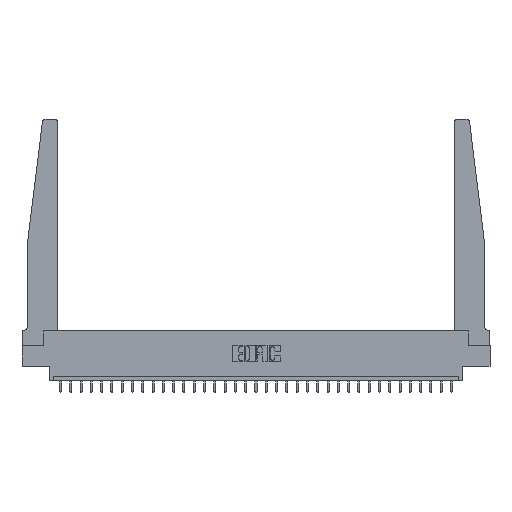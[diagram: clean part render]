
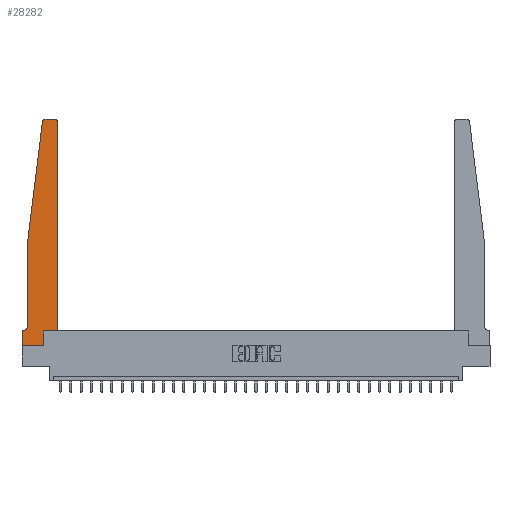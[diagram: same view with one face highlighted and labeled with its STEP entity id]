
A CAD part, top view. The second image highlights one B-rep face of the part: STEP entity #28282.
In plain terms, the highlighted planar face has unit normal (0, 0, 1).
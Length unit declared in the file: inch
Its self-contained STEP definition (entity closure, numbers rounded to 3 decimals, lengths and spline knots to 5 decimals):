
#91 = AXIS2_PLACEMENT_3D ( 'NONE', #8846, #29325, #2032 ) ;
#441 = VECTOR ( 'NONE', #27122, 39.37008 ) ;
#779 = CARTESIAN_POINT ( 'NONE',  ( 0.065, 0.1875, 0.37 ) ) ;
#1019 = CARTESIAN_POINT ( 'NONE',  ( 0., 0., 0.37 ) ) ;
#1535 = EDGE_CURVE ( 'NONE', #14042, #28770, #10445, .T. ) ;
#1689 = CIRCLE ( 'NONE', #91, 0.03 ) ;
#1953 = CARTESIAN_POINT ( 'NONE',  ( 0.395, 2.75, 0.37 ) ) ;
#1977 = VERTEX_POINT ( 'NONE', #6697 ) ;
#2004 = DIRECTION ( 'NONE',  ( 0., 0., 1. ) ) ;
#2032 = DIRECTION ( 'NONE',  ( 1., 0., 0. ) ) ;
#2350 = ORIENTED_EDGE ( 'NONE', *, *, #19628, .T. ) ;
#2964 = EDGE_CURVE ( 'NONE', #11977, #5336, #17540, .T. ) ;
#3308 = VECTOR ( 'NONE', #5268, 39.37008 ) ;
#3410 = ORIENTED_EDGE ( 'NONE', *, *, #10364, .T. ) ;
#3587 = CARTESIAN_POINT ( 'NONE',  ( 0., 0.1875, 0.37 ) ) ;
#4598 = ORIENTED_EDGE ( 'NONE', *, *, #2964, .T. ) ;
#4945 = CARTESIAN_POINT ( 'NONE',  ( 0.2605, 0.18, 0.37 ) ) ;
#5031 = DIRECTION ( 'NONE',  ( 0., 1., 0. ) ) ;
#5268 = DIRECTION ( 'NONE',  ( -0.122, -0.992, 0. ) ) ;
#5336 = VERTEX_POINT ( 'NONE', #24754 ) ;
#5900 = CARTESIAN_POINT ( 'NONE',  ( 0.25, 2.75, 0.37 ) ) ;
#6135 = DIRECTION ( 'NONE',  ( 1., 0., 0. ) ) ;
#6365 = VECTOR ( 'NONE', #18837, 39.37008 ) ;
#6383 = FACE_OUTER_BOUND ( 'NONE', #23536, .T. ) ;
#6697 = CARTESIAN_POINT ( 'NONE',  ( 0.065, 0.2375, 0.37 ) ) ;
#6824 = CARTESIAN_POINT ( 'NONE',  ( 0.2605, 0.18, 0.37 ) ) ;
#6876 = ORIENTED_EDGE ( 'NONE', *, *, #23382, .T. ) ;
#8528 = DIRECTION ( 'NONE',  ( 1., 0., 0. ) ) ;
#8624 = EDGE_CURVE ( 'NONE', #1977, #20316, #21127, .T. ) ;
#8846 = CARTESIAN_POINT ( 'NONE',  ( 0.395, 2.72, 0.37 ) ) ;
#9154 = AXIS2_PLACEMENT_3D ( 'NONE', #10715, #23540, #12093 ) ;
#9339 = ORIENTED_EDGE ( 'NONE', *, *, #8624, .T. ) ;
#9662 = CARTESIAN_POINT ( 'NONE',  ( 0.24675, 2.72367, 0.37 ) ) ;
#10057 = LINE ( 'NONE', #4945, #19785 ) ;
#10078 = ORIENTED_EDGE ( 'NONE', *, *, #23484, .T. ) ;
#10087 = CARTESIAN_POINT ( 'NONE',  ( 0.425, 2.72, 0.37 ) ) ;
#10134 = CARTESIAN_POINT ( 'NONE',  ( 0.425, 0.18, 0.37 ) ) ;
#10364 = EDGE_CURVE ( 'NONE', #13816, #14042, #1689, .T. ) ;
#10445 = LINE ( 'NONE', #5900, #19095 ) ;
#10715 = CARTESIAN_POINT ( 'NONE',  ( 0.015, 0.2375, 0.37 ) ) ;
#11278 = VERTEX_POINT ( 'NONE', #1019 ) ;
#11977 = VERTEX_POINT ( 'NONE', #6824 ) ;
#12093 = DIRECTION ( 'NONE',  ( -1., 0., 0. ) ) ;
#12446 = EDGE_CURVE ( 'NONE', #28100, #11977, #10057, .T. ) ;
#12649 = ORIENTED_EDGE ( 'NONE', *, *, #12976, .T. ) ;
#12976 = EDGE_CURVE ( 'NONE', #28484, #15863, #16868, .T. ) ;
#13419 = CARTESIAN_POINT ( 'NONE',  ( 0.065, 1.25, 0.37 ) ) ;
#13816 = VERTEX_POINT ( 'NONE', #10087 ) ;
#14042 = VERTEX_POINT ( 'NONE', #1953 ) ;
#14852 = DIRECTION ( 'NONE',  ( -1., 0., 0. ) ) ;
#14882 = ORIENTED_EDGE ( 'NONE', *, *, #12446, .T. ) ;
#15025 = VECTOR ( 'NONE', #29393, 39.37008 ) ;
#15396 = ORIENTED_EDGE ( 'NONE', *, *, #1535, .T. ) ;
#15401 = CARTESIAN_POINT ( 'NONE',  ( 0., 0., 0.37 ) ) ;
#15425 = CIRCLE ( 'NONE', #27585, 0.03 ) ;
#15863 = VERTEX_POINT ( 'NONE', #16397 ) ;
#16135 = DIRECTION ( 'NONE',  ( 0., 1., 0. ) ) ;
#16397 = CARTESIAN_POINT ( 'NONE',  ( 0.065, 1.25, 0.37 ) ) ;
#16417 = DIRECTION ( 'NONE',  ( 1., 0., 0. ) ) ;
#16868 = LINE ( 'NONE', #18656, #3308 ) ;
#17015 = VECTOR ( 'NONE', #8528, 39.37008 ) ;
#17228 = DIRECTION ( 'NONE',  ( 0., -1., 0. ) ) ;
#17294 = CARTESIAN_POINT ( 'NONE',  ( 0.27653, 2.72, 0.37 ) ) ;
#17540 = LINE ( 'NONE', #10134, #441 ) ;
#18656 = CARTESIAN_POINT ( 'NONE',  ( 0.065, 1.25, 0.37 ) ) ;
#18837 = DIRECTION ( 'NONE',  ( -1., 0., 0. ) ) ;
#19095 = VECTOR ( 'NONE', #14852, 39.37008 ) ;
#19363 = LINE ( 'NONE', #13419, #15025 ) ;
#19628 = EDGE_CURVE ( 'NONE', #11278, #28100, #23099, .T. ) ;
#19785 = VECTOR ( 'NONE', #5031, 39.37008 ) ;
#19822 = DIRECTION ( 'NONE',  ( 0., 0., 1. ) ) ;
#19944 = LINE ( 'NONE', #779, #6365 ) ;
#20074 = VECTOR ( 'NONE', #16135, 39.37008 ) ;
#20129 = CARTESIAN_POINT ( 'NONE',  ( 0.015, 0.1875, 0.37 ) ) ;
#20182 = CARTESIAN_POINT ( 'NONE',  ( 0., 0.1875, 0.37 ) ) ;
#20316 = VERTEX_POINT ( 'NONE', #20129 ) ;
#21127 = CIRCLE ( 'NONE', #9154, 0.05 ) ;
#21854 = CARTESIAN_POINT ( 'NONE',  ( 0., 0., 0.37 ) ) ;
#22189 = VECTOR ( 'NONE', #17228, 39.37008 ) ;
#22659 = EDGE_CURVE ( 'NONE', #28770, #28484, #15425, .T. ) ;
#22677 = ORIENTED_EDGE ( 'NONE', *, *, #22659, .T. ) ;
#23099 = LINE ( 'NONE', #15401, #17015 ) ;
#23382 = EDGE_CURVE ( 'NONE', #15863, #1977, #19363, .T. ) ;
#23439 = ORIENTED_EDGE ( 'NONE', *, *, #23805, .T. ) ;
#23484 = EDGE_CURVE ( 'NONE', #5336, #13816, #23653, .T. ) ;
#23519 = CARTESIAN_POINT ( 'NONE',  ( 0.2605, 0., 0.37 ) ) ;
#23536 = EDGE_LOOP ( 'NONE', ( #15396, #22677, #12649, #6876, #9339, #28319, #23439, #2350, #14882, #4598, #10078, #3410 ) ) ;
#23540 = DIRECTION ( 'NONE',  ( 0., 0., -1. ) ) ;
#23653 = LINE ( 'NONE', #25451, #20074 ) ;
#23805 = EDGE_CURVE ( 'NONE', #27653, #11278, #28226, .T. ) ;
#24754 = CARTESIAN_POINT ( 'NONE',  ( 0.425, 0.18, 0.37 ) ) ;
#25451 = CARTESIAN_POINT ( 'NONE',  ( 0.425, 0.18, 0.37 ) ) ;
#25800 = PLANE ( 'NONE',  #29022 ) ;
#26289 = EDGE_CURVE ( 'NONE', #20316, #27653, #19944, .T. ) ;
#26395 = CARTESIAN_POINT ( 'NONE',  ( 0.27653, 2.75, 0.37 ) ) ;
#27122 = DIRECTION ( 'NONE',  ( 1., 0., 0. ) ) ;
#27585 = AXIS2_PLACEMENT_3D ( 'NONE', #17294, #19822, #6135 ) ;
#27653 = VERTEX_POINT ( 'NONE', #3587 ) ;
#28100 = VERTEX_POINT ( 'NONE', #23519 ) ;
#28226 = LINE ( 'NONE', #21854, #22189 ) ;
#28282 = ADVANCED_FACE ( 'NONE', ( #6383 ), #25800, .T. ) ;
#28319 = ORIENTED_EDGE ( 'NONE', *, *, #26289, .T. ) ;
#28484 = VERTEX_POINT ( 'NONE', #9662 ) ;
#28770 = VERTEX_POINT ( 'NONE', #26395 ) ;
#29022 = AXIS2_PLACEMENT_3D ( 'NONE', #20182, #2004, #16417 ) ;
#29325 = DIRECTION ( 'NONE',  ( 0., 0., 1. ) ) ;
#29393 = DIRECTION ( 'NONE',  ( 0., -1., 0. ) ) ;
